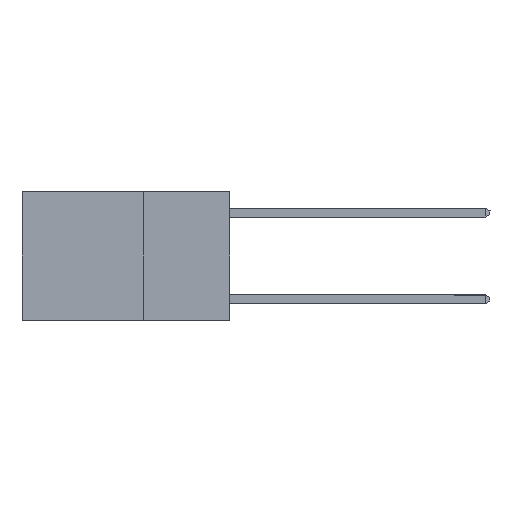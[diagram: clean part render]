
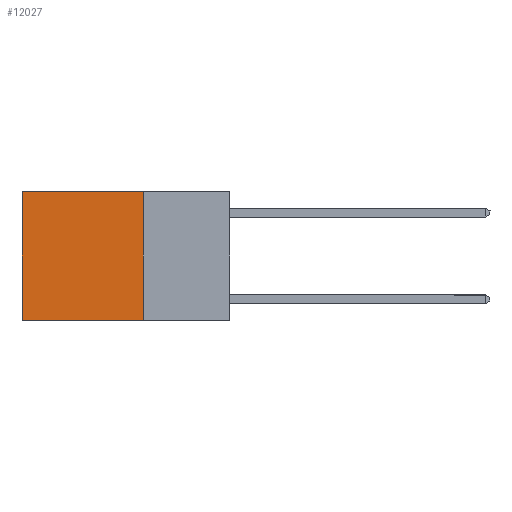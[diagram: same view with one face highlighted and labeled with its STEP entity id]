
A CAD part, left-side view. The second image highlights one B-rep face of the part: STEP entity #12027.
In plain terms, the highlighted planar face has unit normal (-1, 0, 0).
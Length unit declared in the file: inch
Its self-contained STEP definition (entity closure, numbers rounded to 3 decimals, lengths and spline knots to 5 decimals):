
#1758 = EDGE_CURVE ( 'NONE', #13296, #5633, #21834, .T. ) ;
#2501 = LINE ( 'NONE', #10188, #21373 ) ;
#2709 = VERTEX_POINT ( 'NONE', #22088 ) ;
#2931 = DIRECTION ( 'NONE',  ( 1., 0., 0. ) ) ;
#3838 = EDGE_CURVE ( 'NONE', #13296, #18959, #14978, .T. ) ;
#4211 = AXIS2_PLACEMENT_3D ( 'NONE', #10382, #2931, #16115 ) ;
#4540 = ORIENTED_EDGE ( 'NONE', *, *, #7034, .F. ) ;
#5564 = VECTOR ( 'NONE', #10506, 39.37008 ) ;
#5633 = VERTEX_POINT ( 'NONE', #8277 ) ;
#6018 = CARTESIAN_POINT ( 'NONE',  ( 0.2625, 0.25, 0. ) ) ;
#7034 = EDGE_CURVE ( 'NONE', #18959, #2709, #2501, .T. ) ;
#7870 = DIRECTION ( 'NONE',  ( 0., 1., 0. ) ) ;
#8277 = CARTESIAN_POINT ( 'NONE',  ( 0.2625, 0.6, 0. ) ) ;
#9232 = ORIENTED_EDGE ( 'NONE', *, *, #3838, .F. ) ;
#9769 = LINE ( 'NONE', #16613, #13608 ) ;
#10188 = CARTESIAN_POINT ( 'NONE',  ( 0.2625, 0.25, -0.37 ) ) ;
#10382 = CARTESIAN_POINT ( 'NONE',  ( 0.2625, 0.25, 0. ) ) ;
#10506 = DIRECTION ( 'NONE',  ( 0., 0., -1. ) ) ;
#11731 = VECTOR ( 'NONE', #7870, 39.37008 ) ;
#12027 = ADVANCED_FACE ( 'NONE', ( #15917 ), #14198, .F. ) ;
#12072 = DIRECTION ( 'NONE',  ( 0., 1., 0. ) ) ;
#12316 = CARTESIAN_POINT ( 'NONE',  ( 0.2625, 0.25, 0. ) ) ;
#13296 = VERTEX_POINT ( 'NONE', #12316 ) ;
#13608 = VECTOR ( 'NONE', #18504, 39.37008 ) ;
#14198 = PLANE ( 'NONE',  #4211 ) ;
#14978 = LINE ( 'NONE', #21870, #5564 ) ;
#15283 = CARTESIAN_POINT ( 'NONE',  ( 0.2625, 0.25, -0.37 ) ) ;
#15917 = FACE_OUTER_BOUND ( 'NONE', #22183, .T. ) ;
#15922 = ORIENTED_EDGE ( 'NONE', *, *, #1758, .T. ) ;
#16115 = DIRECTION ( 'NONE',  ( 0., 0., -1. ) ) ;
#16401 = ORIENTED_EDGE ( 'NONE', *, *, #16813, .T. ) ;
#16613 = CARTESIAN_POINT ( 'NONE',  ( 0.2625, 0.6, 0. ) ) ;
#16813 = EDGE_CURVE ( 'NONE', #5633, #2709, #9769, .T. ) ;
#18504 = DIRECTION ( 'NONE',  ( 0., 0., -1. ) ) ;
#18959 = VERTEX_POINT ( 'NONE', #15283 ) ;
#21373 = VECTOR ( 'NONE', #12072, 39.37008 ) ;
#21834 = LINE ( 'NONE', #6018, #11731 ) ;
#21870 = CARTESIAN_POINT ( 'NONE',  ( 0.2625, 0.25, 0. ) ) ;
#22088 = CARTESIAN_POINT ( 'NONE',  ( 0.2625, 0.6, -0.37 ) ) ;
#22183 = EDGE_LOOP ( 'NONE', ( #16401, #4540, #9232, #15922 ) ) ;
